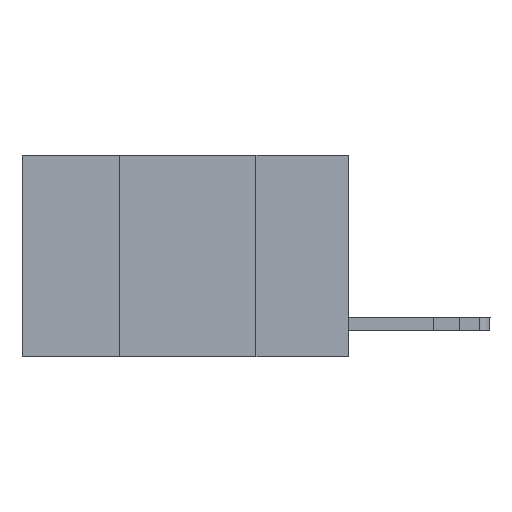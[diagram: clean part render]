
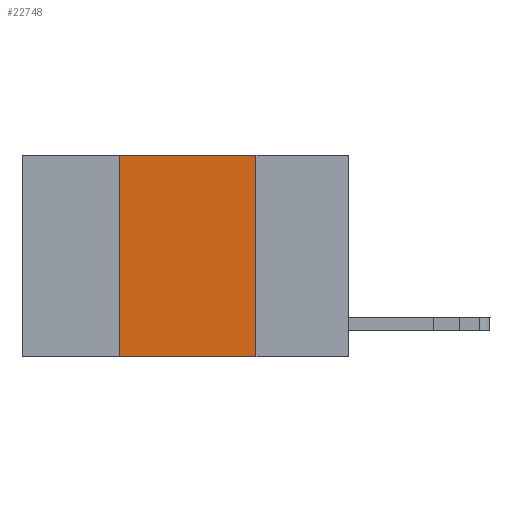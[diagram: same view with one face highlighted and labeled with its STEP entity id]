
A CAD part, left-side view. The second image highlights one B-rep face of the part: STEP entity #22748.
In plain terms, the highlighted planar face has unit normal (-1, 0, 0).
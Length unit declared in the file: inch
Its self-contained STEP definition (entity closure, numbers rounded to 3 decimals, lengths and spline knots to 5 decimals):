
#164 = EDGE_LOOP ( 'NONE', ( #21571, #21542, #3466, #4856 ) ) ;
#3420 = VECTOR ( 'NONE', #3865, 39.37008 ) ;
#3466 = ORIENTED_EDGE ( 'NONE', *, *, #8234, .F. ) ;
#3539 = VECTOR ( 'NONE', #25243, 39.37008 ) ;
#3688 = LINE ( 'NONE', #21378, #3539 ) ;
#3865 = DIRECTION ( 'NONE',  ( 0., 0., 1. ) ) ;
#4239 = CARTESIAN_POINT ( 'NONE',  ( 0., 0.6, -0.37 ) ) ;
#4856 = ORIENTED_EDGE ( 'NONE', *, *, #6940, .T. ) ;
#5402 = EDGE_CURVE ( 'NONE', #22570, #13423, #3688, .T. ) ;
#5793 = LINE ( 'NONE', #21664, #3420 ) ;
#6173 = LINE ( 'NONE', #4239, #20366 ) ;
#6940 = EDGE_CURVE ( 'NONE', #14771, #16828, #6173, .T. ) ;
#7220 = AXIS2_PLACEMENT_3D ( 'NONE', #9208, #21030, #10756 ) ;
#7910 = EDGE_CURVE ( 'NONE', #13423, #16828, #12576, .T. ) ;
#8234 = EDGE_CURVE ( 'NONE', #14771, #22570, #5793, .T. ) ;
#9208 = CARTESIAN_POINT ( 'NONE',  ( 0., 0.6, 0. ) ) ;
#10636 = CARTESIAN_POINT ( 'NONE',  ( 0., 0.42, 0. ) ) ;
#10756 = DIRECTION ( 'NONE',  ( 0., 0., -1. ) ) ;
#12245 = CARTESIAN_POINT ( 'NONE',  ( 0., 0.17, -0.37 ) ) ;
#12576 = LINE ( 'NONE', #16755, #20403 ) ;
#12836 = DIRECTION ( 'NONE',  ( 0., 0., -1. ) ) ;
#13423 = VERTEX_POINT ( 'NONE', #19689 ) ;
#14771 = VERTEX_POINT ( 'NONE', #16153 ) ;
#15576 = DIRECTION ( 'NONE',  ( 0., -1., 0. ) ) ;
#16153 = CARTESIAN_POINT ( 'NONE',  ( 0., 0.42, -0.37 ) ) ;
#16755 = CARTESIAN_POINT ( 'NONE',  ( 0., 0.17, 0. ) ) ;
#16828 = VERTEX_POINT ( 'NONE', #12245 ) ;
#18975 = PLANE ( 'NONE',  #7220 ) ;
#19689 = CARTESIAN_POINT ( 'NONE',  ( 0., 0.17, 0. ) ) ;
#20366 = VECTOR ( 'NONE', #15576, 39.37008 ) ;
#20403 = VECTOR ( 'NONE', #12836, 39.37008 ) ;
#21030 = DIRECTION ( 'NONE',  ( 1., 0., 0. ) ) ;
#21286 = FACE_OUTER_BOUND ( 'NONE', #164, .T. ) ;
#21378 = CARTESIAN_POINT ( 'NONE',  ( 0., 0.6, 0. ) ) ;
#21542 = ORIENTED_EDGE ( 'NONE', *, *, #5402, .F. ) ;
#21571 = ORIENTED_EDGE ( 'NONE', *, *, #7910, .F. ) ;
#21664 = CARTESIAN_POINT ( 'NONE',  ( 0., 0.42, 0. ) ) ;
#22570 = VERTEX_POINT ( 'NONE', #10636 ) ;
#22748 = ADVANCED_FACE ( 'NONE', ( #21286 ), #18975, .F. ) ;
#25243 = DIRECTION ( 'NONE',  ( 0., -1., 0. ) ) ;
